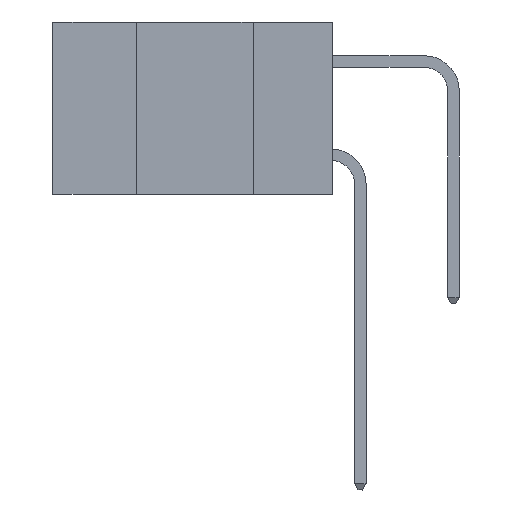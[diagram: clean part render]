
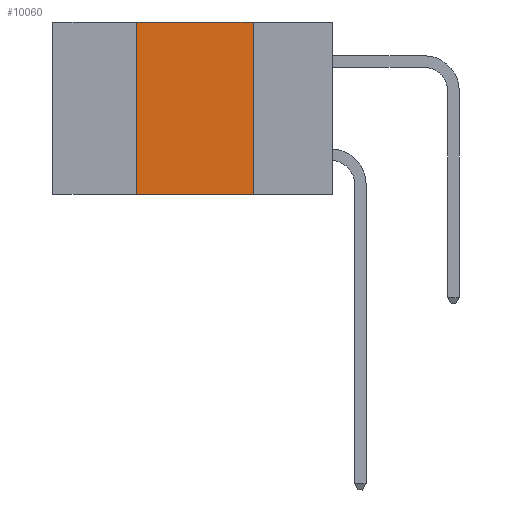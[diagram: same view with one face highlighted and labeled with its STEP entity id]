
A CAD part, left-side view. The second image highlights one B-rep face of the part: STEP entity #10060.
In plain terms, the highlighted planar face has unit normal (-1, 0, 0).
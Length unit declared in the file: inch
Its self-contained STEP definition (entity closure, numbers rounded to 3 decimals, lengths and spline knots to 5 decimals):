
#137 = CARTESIAN_POINT ( 'NONE',  ( 0., 0.17, 0. ) ) ;
#544 = LINE ( 'NONE', #6875, #5135 ) ;
#602 = EDGE_CURVE ( 'NONE', #2278, #1155, #5028, .T. ) ;
#804 = PLANE ( 'NONE',  #9612 ) ;
#1155 = VERTEX_POINT ( 'NONE', #7515 ) ;
#1218 = EDGE_LOOP ( 'NONE', ( #13132, #4794, #1654, #3271 ) ) ;
#1461 = EDGE_CURVE ( 'NONE', #8996, #1155, #5001, .T. ) ;
#1631 = CARTESIAN_POINT ( 'NONE',  ( 0., 0.6, -0.37 ) ) ;
#1654 = ORIENTED_EDGE ( 'NONE', *, *, #3072, .F. ) ;
#1674 = EDGE_CURVE ( 'NONE', #13235, #8996, #8424, .T. ) ;
#1853 = DIRECTION ( 'NONE',  ( 0., 0., -1. ) ) ;
#2220 = VECTOR ( 'NONE', #8735, 39.37008 ) ;
#2278 = VERTEX_POINT ( 'NONE', #9706 ) ;
#3072 = EDGE_CURVE ( 'NONE', #2278, #13235, #544, .T. ) ;
#3271 = ORIENTED_EDGE ( 'NONE', *, *, #602, .T. ) ;
#3820 = FACE_OUTER_BOUND ( 'NONE', #1218, .T. ) ;
#3938 = CARTESIAN_POINT ( 'NONE',  ( 0., 0.6, 0. ) ) ;
#4794 = ORIENTED_EDGE ( 'NONE', *, *, #1674, .F. ) ;
#5001 = LINE ( 'NONE', #12459, #13191 ) ;
#5028 = LINE ( 'NONE', #1631, #2220 ) ;
#5135 = VECTOR ( 'NONE', #9291, 39.37008 ) ;
#6219 = DIRECTION ( 'NONE',  ( 0., -1., 0. ) ) ;
#6875 = CARTESIAN_POINT ( 'NONE',  ( 0., 0.42, 0. ) ) ;
#7515 = CARTESIAN_POINT ( 'NONE',  ( 0., 0.17, -0.37 ) ) ;
#8283 = DIRECTION ( 'NONE',  ( 1., 0., 0. ) ) ;
#8424 = LINE ( 'NONE', #13042, #10915 ) ;
#8735 = DIRECTION ( 'NONE',  ( 0., -1., 0. ) ) ;
#8996 = VERTEX_POINT ( 'NONE', #137 ) ;
#9291 = DIRECTION ( 'NONE',  ( 0., 0., 1. ) ) ;
#9612 = AXIS2_PLACEMENT_3D ( 'NONE', #3938, #8283, #1853 ) ;
#9706 = CARTESIAN_POINT ( 'NONE',  ( 0., 0.42, -0.37 ) ) ;
#10018 = CARTESIAN_POINT ( 'NONE',  ( 0., 0.42, 0. ) ) ;
#10060 = ADVANCED_FACE ( 'NONE', ( #3820 ), #804, .F. ) ;
#10915 = VECTOR ( 'NONE', #6219, 39.37008 ) ;
#11129 = DIRECTION ( 'NONE',  ( 0., 0., -1. ) ) ;
#12459 = CARTESIAN_POINT ( 'NONE',  ( 0., 0.17, 0. ) ) ;
#13042 = CARTESIAN_POINT ( 'NONE',  ( 0., 0.6, 0. ) ) ;
#13132 = ORIENTED_EDGE ( 'NONE', *, *, #1461, .F. ) ;
#13191 = VECTOR ( 'NONE', #11129, 39.37008 ) ;
#13235 = VERTEX_POINT ( 'NONE', #10018 ) ;
